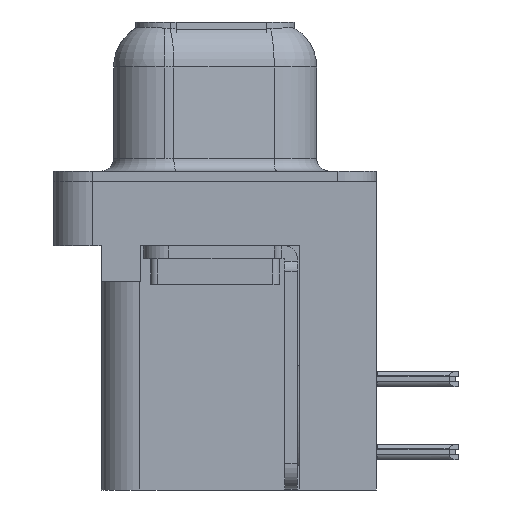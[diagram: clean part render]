
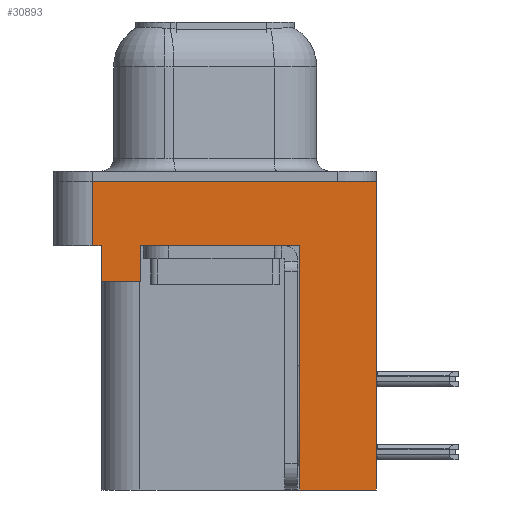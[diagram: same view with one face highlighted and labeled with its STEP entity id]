
A CAD part, left-side view. The second image highlights one B-rep face of the part: STEP entity #30893.
In plain terms, the highlighted planar face has unit normal (-1, 0, 0).
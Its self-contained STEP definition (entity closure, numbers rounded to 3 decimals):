
#581 = LINE ( 'NONE', #2316, #14466 ) ;
#1310 = DIRECTION ( 'NONE',  ( 0., -1., 0. ) ) ;
#1335 = ORIENTED_EDGE ( 'NONE', *, *, #2472, .F. ) ;
#1636 = FACE_OUTER_BOUND ( 'NONE', #17264, .T. ) ;
#1996 = DIRECTION ( 'NONE',  ( 0., 0., 1. ) ) ;
#2137 = EDGE_CURVE ( 'NONE', #21642, #20578, #32306, .T. ) ;
#2316 = CARTESIAN_POINT ( 'NONE',  ( -3., 4.775, -2.5 ) ) ;
#2472 = EDGE_CURVE ( 'NONE', #31990, #18584, #31094, .T. ) ;
#2687 = CARTESIAN_POINT ( 'NONE',  ( -3., 2.895, -3.9 ) ) ;
#3110 = EDGE_CURVE ( 'NONE', #20578, #25818, #25885, .T. ) ;
#3146 = DIRECTION ( 'NONE',  ( 0., -1., 0. ) ) ;
#4379 = DIRECTION ( 'NONE',  ( -1., 0., 0. ) ) ;
#4636 = DIRECTION ( 'NONE',  ( 0., 0., 1. ) ) ;
#4820 = CARTESIAN_POINT ( 'NONE',  ( -3., -6.275, -2.5 ) ) ;
#4835 = LINE ( 'NONE', #4820, #17584 ) ;
#4926 = DIRECTION ( 'NONE',  ( 0., 0., 1. ) ) ;
#6243 = EDGE_CURVE ( 'NONE', #28138, #14376, #19470, .T. ) ;
#6344 = VERTEX_POINT ( 'NONE', #18820 ) ;
#7722 = CARTESIAN_POINT ( 'NONE',  ( -3., -3.295, -12. ) ) ;
#7781 = ORIENTED_EDGE ( 'NONE', *, *, #20210, .F. ) ;
#7912 = CARTESIAN_POINT ( 'NONE',  ( -3., -6.275, 0. ) ) ;
#8705 = EDGE_CURVE ( 'NONE', #6344, #28138, #581, .T. ) ;
#8951 = CARTESIAN_POINT ( 'NONE',  ( -3., -6.275, -12. ) ) ;
#11113 = VECTOR ( 'NONE', #3146, 1000. ) ;
#11614 = ORIENTED_EDGE ( 'NONE', *, *, #3110, .F. ) ;
#11972 = DIRECTION ( 'NONE',  ( 0., 0., 1. ) ) ;
#13775 = CARTESIAN_POINT ( 'NONE',  ( -3., 4.775, 0. ) ) ;
#14039 = CARTESIAN_POINT ( 'NONE',  ( -3., -6.275, -2.5 ) ) ;
#14158 = ORIENTED_EDGE ( 'NONE', *, *, #2137, .F. ) ;
#14376 = VERTEX_POINT ( 'NONE', #23326 ) ;
#14466 = VECTOR ( 'NONE', #4636, 1000. ) ;
#15361 = EDGE_CURVE ( 'NONE', #31450, #25818, #25883, .T. ) ;
#16136 = CARTESIAN_POINT ( 'NONE',  ( -3., -3.295, -2.5 ) ) ;
#16250 = VERTEX_POINT ( 'NONE', #2687 ) ;
#16750 = VECTOR ( 'NONE', #1310, 1000. ) ;
#16802 = LINE ( 'NONE', #14039, #26740 ) ;
#16961 = DIRECTION ( 'NONE',  ( 0., 0., 1. ) ) ;
#17157 = VECTOR ( 'NONE', #1996, 1000. ) ;
#17264 = EDGE_LOOP ( 'NONE', ( #29227, #24178, #32432, #1335, #7781, #25330, #23445, #11614, #14158, #26283 ) ) ;
#17584 = VECTOR ( 'NONE', #4926, 1000. ) ;
#18584 = VERTEX_POINT ( 'NONE', #30014 ) ;
#18702 = EDGE_CURVE ( 'NONE', #6344, #18584, #16802, .T. ) ;
#18820 = CARTESIAN_POINT ( 'NONE',  ( -3., 4.775, -2.5 ) ) ;
#18987 = CARTESIAN_POINT ( 'NONE',  ( -3., -6.275, -2.5 ) ) ;
#19225 = DIRECTION ( 'NONE',  ( 0., 0., 1. ) ) ;
#19337 = CARTESIAN_POINT ( 'NONE',  ( -3., 4.425, -3.9 ) ) ;
#19470 = LINE ( 'NONE', #7912, #11113 ) ;
#20210 = EDGE_CURVE ( 'NONE', #16250, #31990, #23876, .T. ) ;
#20426 = VECTOR ( 'NONE', #16961, 1000. ) ;
#20578 = VERTEX_POINT ( 'NONE', #7722 ) ;
#21642 = VERTEX_POINT ( 'NONE', #8951 ) ;
#22395 = VECTOR ( 'NONE', #19225, 1000. ) ;
#23326 = CARTESIAN_POINT ( 'NONE',  ( -3., -6.275, 0. ) ) ;
#23445 = ORIENTED_EDGE ( 'NONE', *, *, #15361, .T. ) ;
#23876 = LINE ( 'NONE', #24694, #25427 ) ;
#24068 = CARTESIAN_POINT ( 'NONE',  ( -3., -6.275, -2.5 ) ) ;
#24102 = CARTESIAN_POINT ( 'NONE',  ( -3., 2.895, -3.9 ) ) ;
#24178 = ORIENTED_EDGE ( 'NONE', *, *, #8705, .F. ) ;
#24476 = DIRECTION ( 'NONE',  ( 0., 1., 0. ) ) ;
#24694 = CARTESIAN_POINT ( 'NONE',  ( -3., 4.425, -3.9 ) ) ;
#25307 = EDGE_CURVE ( 'NONE', #16250, #31450, #27541, .T. ) ;
#25330 = ORIENTED_EDGE ( 'NONE', *, *, #25307, .T. ) ;
#25427 = VECTOR ( 'NONE', #24476, 1000. ) ;
#25818 = VERTEX_POINT ( 'NONE', #16136 ) ;
#25883 = LINE ( 'NONE', #18987, #16750 ) ;
#25885 = LINE ( 'NONE', #32392, #17157 ) ;
#26283 = ORIENTED_EDGE ( 'NONE', *, *, #26401, .T. ) ;
#26401 = EDGE_CURVE ( 'NONE', #21642, #14376, #4835, .T. ) ;
#26502 = AXIS2_PLACEMENT_3D ( 'NONE', #24068, #4379, #11972 ) ;
#26740 = VECTOR ( 'NONE', #31562, 1000. ) ;
#27035 = PLANE ( 'NONE',  #26502 ) ;
#27450 = CARTESIAN_POINT ( 'NONE',  ( -3., 2.895, -2.5 ) ) ;
#27541 = LINE ( 'NONE', #24102, #22395 ) ;
#28138 = VERTEX_POINT ( 'NONE', #13775 ) ;
#28740 = VECTOR ( 'NONE', #31882, 1000. ) ;
#29227 = ORIENTED_EDGE ( 'NONE', *, *, #6243, .F. ) ;
#29664 = CARTESIAN_POINT ( 'NONE',  ( -3., -3.295, -12. ) ) ;
#30014 = CARTESIAN_POINT ( 'NONE',  ( -3., 4.425, -2.5 ) ) ;
#30893 = ADVANCED_FACE ( 'NONE', ( #1636 ), #27035, .T. ) ;
#31094 = LINE ( 'NONE', #19337, #20426 ) ;
#31450 = VERTEX_POINT ( 'NONE', #27450 ) ;
#31562 = DIRECTION ( 'NONE',  ( 0., -1., 0. ) ) ;
#31882 = DIRECTION ( 'NONE',  ( 0., 1., 0. ) ) ;
#31990 = VERTEX_POINT ( 'NONE', #32522 ) ;
#32306 = LINE ( 'NONE', #29664, #28740 ) ;
#32392 = CARTESIAN_POINT ( 'NONE',  ( -3., -3.295, -12. ) ) ;
#32432 = ORIENTED_EDGE ( 'NONE', *, *, #18702, .T. ) ;
#32522 = CARTESIAN_POINT ( 'NONE',  ( -3., 4.425, -3.9 ) ) ;
